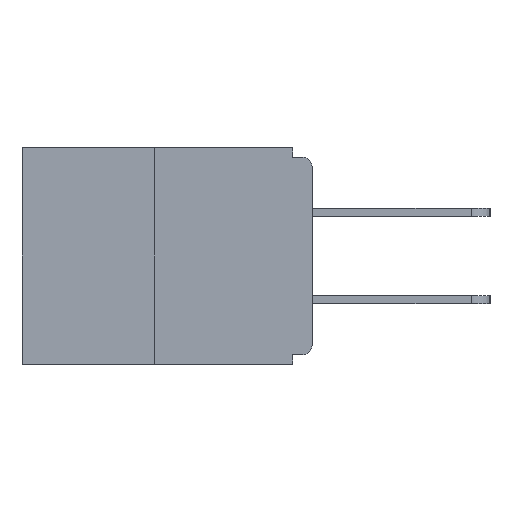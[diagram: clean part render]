
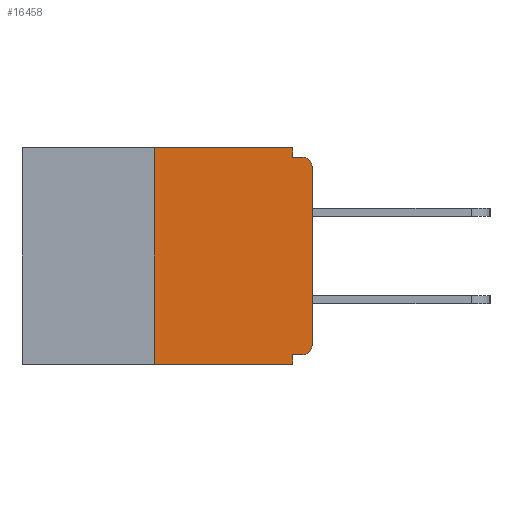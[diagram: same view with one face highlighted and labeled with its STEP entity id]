
A CAD part, left-side view. The second image highlights one B-rep face of the part: STEP entity #16458.
In plain terms, the highlighted planar face has unit normal (-1, 0, 0).
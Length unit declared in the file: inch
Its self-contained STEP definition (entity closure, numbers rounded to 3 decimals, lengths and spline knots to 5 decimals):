
#126 = ORIENTED_EDGE ( 'NONE', *, *, #5017, .T. ) ;
#448 = AXIS2_PLACEMENT_3D ( 'NONE', #9936, #11261, #6939 ) ;
#584 = VERTEX_POINT ( 'NONE', #2328 ) ;
#796 = CARTESIAN_POINT ( 'NONE',  ( 0., 0., 0. ) ) ;
#915 = CARTESIAN_POINT ( 'NONE',  ( 0., 0.25, 0. ) ) ;
#1110 = CIRCLE ( 'NONE', #14553, 0.015 ) ;
#1796 = ORIENTED_EDGE ( 'NONE', *, *, #18395, .F. ) ;
#2033 = CARTESIAN_POINT ( 'NONE',  ( 0., 0.015, -0.328 ) ) ;
#2229 = LINE ( 'NONE', #2726, #13200 ) ;
#2328 = CARTESIAN_POINT ( 'NONE',  ( 0., 0., -0.313 ) ) ;
#2645 = ORIENTED_EDGE ( 'NONE', *, *, #9881, .F. ) ;
#2726 = CARTESIAN_POINT ( 'NONE',  ( 0., 0.46, -0.343 ) ) ;
#2942 = LINE ( 'NONE', #14878, #12236 ) ;
#2958 = VERTEX_POINT ( 'NONE', #19340 ) ;
#3509 = CARTESIAN_POINT ( 'NONE',  ( 0., 0., -0.03 ) ) ;
#3537 = VERTEX_POINT ( 'NONE', #16483 ) ;
#3549 = VECTOR ( 'NONE', #8761, 39.37008 ) ;
#3836 = CARTESIAN_POINT ( 'NONE',  ( 0., 0.46, 0. ) ) ;
#4575 = VERTEX_POINT ( 'NONE', #9918 ) ;
#4792 = LINE ( 'NONE', #796, #16713 ) ;
#5017 = EDGE_CURVE ( 'NONE', #5133, #2958, #1110, .T. ) ;
#5133 = VERTEX_POINT ( 'NONE', #3509 ) ;
#5392 = EDGE_CURVE ( 'NONE', #13428, #4575, #9195, .T. ) ;
#5457 = CARTESIAN_POINT ( 'NONE',  ( 0., 0.46, 0. ) ) ;
#5746 = VERTEX_POINT ( 'NONE', #915 ) ;
#6209 = CARTESIAN_POINT ( 'NONE',  ( 0., 0.25, -0.343 ) ) ;
#6331 = ORIENTED_EDGE ( 'NONE', *, *, #6808, .F. ) ;
#6492 = ORIENTED_EDGE ( 'NONE', *, *, #8209, .T. ) ;
#6661 = EDGE_CURVE ( 'NONE', #5746, #3537, #11275, .T. ) ;
#6730 = LINE ( 'NONE', #16599, #8156 ) ;
#6745 = EDGE_CURVE ( 'NONE', #12132, #4575, #2229, .T. ) ;
#6808 = EDGE_CURVE ( 'NONE', #12132, #5746, #2942, .T. ) ;
#6939 = DIRECTION ( 'NONE',  ( 0., 0., -1. ) ) ;
#7498 = CIRCLE ( 'NONE', #448, 0.015 ) ;
#8156 = VECTOR ( 'NONE', #10507, 39.37008 ) ;
#8209 = EDGE_CURVE ( 'NONE', #584, #5133, #4792, .T. ) ;
#8319 = EDGE_CURVE ( 'NONE', #3537, #15919, #15548, .T. ) ;
#8494 = DIRECTION ( 'NONE',  ( 0., 0., -1. ) ) ;
#8761 = DIRECTION ( 'NONE',  ( 0., -1., 0. ) ) ;
#8769 = DIRECTION ( 'NONE',  ( 0., 0., 1. ) ) ;
#9195 = LINE ( 'NONE', #13593, #19487 ) ;
#9293 = CARTESIAN_POINT ( 'NONE',  ( 0., 0.031, -0.328 ) ) ;
#9423 = ORIENTED_EDGE ( 'NONE', *, *, #8319, .F. ) ;
#9544 = VECTOR ( 'NONE', #17680, 39.37008 ) ;
#9881 = EDGE_CURVE ( 'NONE', #15919, #2958, #17641, .T. ) ;
#9918 = CARTESIAN_POINT ( 'NONE',  ( 0., 0.031, -0.343 ) ) ;
#9936 = CARTESIAN_POINT ( 'NONE',  ( 0., 0.015, -0.313 ) ) ;
#10214 = PLANE ( 'NONE',  #16444 ) ;
#10236 = DIRECTION ( 'NONE',  ( 0., -1., 0. ) ) ;
#10507 = DIRECTION ( 'NONE',  ( 0., 1., 0. ) ) ;
#11261 = DIRECTION ( 'NONE',  ( -1., 0., 0. ) ) ;
#11275 = LINE ( 'NONE', #5457, #12741 ) ;
#11556 = DIRECTION ( 'NONE',  ( 1., 0., 0. ) ) ;
#11704 = EDGE_CURVE ( 'NONE', #19644, #584, #7498, .T. ) ;
#12132 = VERTEX_POINT ( 'NONE', #6209 ) ;
#12236 = VECTOR ( 'NONE', #8769, 39.37008 ) ;
#12266 = ORIENTED_EDGE ( 'NONE', *, *, #6745, .T. ) ;
#12741 = VECTOR ( 'NONE', #14753, 39.37008 ) ;
#13007 = ORIENTED_EDGE ( 'NONE', *, *, #6661, .F. ) ;
#13112 = CARTESIAN_POINT ( 'NONE',  ( 0., 0.031, -0.015 ) ) ;
#13200 = VECTOR ( 'NONE', #10236, 39.37008 ) ;
#13428 = VERTEX_POINT ( 'NONE', #9293 ) ;
#13593 = CARTESIAN_POINT ( 'NONE',  ( 0., 0.031, -0.343 ) ) ;
#14553 = AXIS2_PLACEMENT_3D ( 'NONE', #14933, #19667, #18072 ) ;
#14753 = DIRECTION ( 'NONE',  ( 0., -1., 0. ) ) ;
#14878 = CARTESIAN_POINT ( 'NONE',  ( 0., 0.25, 0. ) ) ;
#14933 = CARTESIAN_POINT ( 'NONE',  ( 0., 0.015, -0.03 ) ) ;
#15548 = LINE ( 'NONE', #17751, #9544 ) ;
#15919 = VERTEX_POINT ( 'NONE', #13112 ) ;
#16088 = EDGE_LOOP ( 'NONE', ( #13007, #6331, #12266, #16644, #1796, #19294, #6492, #126, #2645, #9423 ) ) ;
#16146 = FACE_OUTER_BOUND ( 'NONE', #16088, .T. ) ;
#16305 = CARTESIAN_POINT ( 'NONE',  ( 0., 0., -0.015 ) ) ;
#16444 = AXIS2_PLACEMENT_3D ( 'NONE', #3836, #11556, #8494 ) ;
#16458 = ADVANCED_FACE ( 'NONE', ( #16146 ), #10214, .F. ) ;
#16483 = CARTESIAN_POINT ( 'NONE',  ( 0., 0.031, 0. ) ) ;
#16599 = CARTESIAN_POINT ( 'NONE',  ( 0., 0., -0.328 ) ) ;
#16644 = ORIENTED_EDGE ( 'NONE', *, *, #5392, .F. ) ;
#16669 = DIRECTION ( 'NONE',  ( 0., 0., -1. ) ) ;
#16713 = VECTOR ( 'NONE', #17484, 39.37008 ) ;
#17484 = DIRECTION ( 'NONE',  ( 0., 0., 1. ) ) ;
#17641 = LINE ( 'NONE', #16305, #3549 ) ;
#17680 = DIRECTION ( 'NONE',  ( 0., 0., -1. ) ) ;
#17751 = CARTESIAN_POINT ( 'NONE',  ( 0., 0.031, 0. ) ) ;
#18072 = DIRECTION ( 'NONE',  ( 0., 0., -1. ) ) ;
#18395 = EDGE_CURVE ( 'NONE', #19644, #13428, #6730, .T. ) ;
#19294 = ORIENTED_EDGE ( 'NONE', *, *, #11704, .T. ) ;
#19340 = CARTESIAN_POINT ( 'NONE',  ( 0., 0.015, -0.015 ) ) ;
#19487 = VECTOR ( 'NONE', #16669, 39.37008 ) ;
#19644 = VERTEX_POINT ( 'NONE', #2033 ) ;
#19667 = DIRECTION ( 'NONE',  ( -1., 0., 0. ) ) ;
